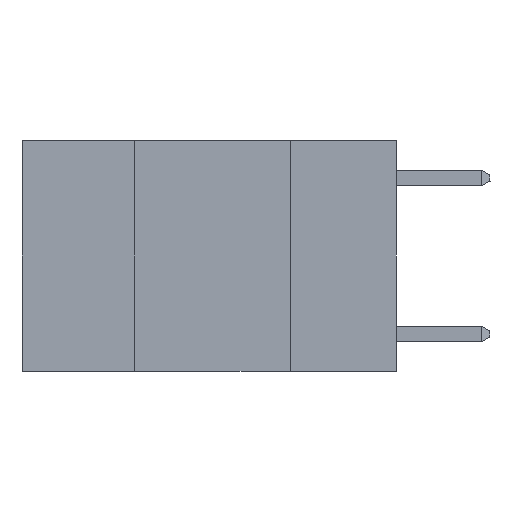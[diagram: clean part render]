
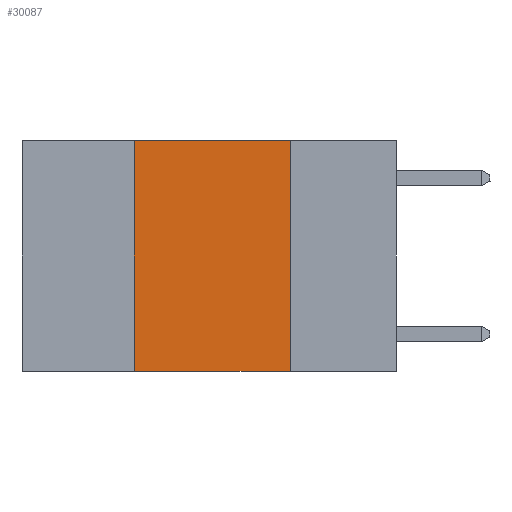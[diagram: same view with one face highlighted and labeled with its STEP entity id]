
A CAD part, left-side view. The second image highlights one B-rep face of the part: STEP entity #30087.
In plain terms, the highlighted planar face has unit normal (-1, 0, 0).
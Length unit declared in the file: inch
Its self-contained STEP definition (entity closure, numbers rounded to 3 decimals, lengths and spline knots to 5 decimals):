
#378 = DIRECTION ( 'NONE',  ( 0., 0., 1. ) ) ;
#1301 = CARTESIAN_POINT ( 'NONE',  ( 0., 0.17, 0. ) ) ;
#1878 = ORIENTED_EDGE ( 'NONE', *, *, #22763, .F. ) ;
#1990 = DIRECTION ( 'NONE',  ( 0., 0., -1. ) ) ;
#2859 = CARTESIAN_POINT ( 'NONE',  ( 0., 0.17, -0.37 ) ) ;
#5022 = CARTESIAN_POINT ( 'NONE',  ( 0., 0.42, 0. ) ) ;
#5112 = VERTEX_POINT ( 'NONE', #1301 ) ;
#5124 = CARTESIAN_POINT ( 'NONE',  ( 0., 0.6, 0. ) ) ;
#5717 = VECTOR ( 'NONE', #8319, 39.37008 ) ;
#6155 = ORIENTED_EDGE ( 'NONE', *, *, #18616, .T. ) ;
#6591 = CARTESIAN_POINT ( 'NONE',  ( 0., 0.6, 0. ) ) ;
#8319 = DIRECTION ( 'NONE',  ( 0., -1., 0. ) ) ;
#8880 = CARTESIAN_POINT ( 'NONE',  ( 0., 0.6, -0.37 ) ) ;
#9042 = VERTEX_POINT ( 'NONE', #2859 ) ;
#10744 = VECTOR ( 'NONE', #1990, 39.37008 ) ;
#12142 = VERTEX_POINT ( 'NONE', #13112 ) ;
#12416 = PLANE ( 'NONE',  #18822 ) ;
#13112 = CARTESIAN_POINT ( 'NONE',  ( 0., 0.42, 0. ) ) ;
#13920 = CARTESIAN_POINT ( 'NONE',  ( 0., 0.17, 0. ) ) ;
#15042 = FACE_OUTER_BOUND ( 'NONE', #21368, .T. ) ;
#15603 = ORIENTED_EDGE ( 'NONE', *, *, #24122, .F. ) ;
#16143 = LINE ( 'NONE', #8880, #29718 ) ;
#18248 = EDGE_CURVE ( 'NONE', #25460, #12142, #24383, .T. ) ;
#18616 = EDGE_CURVE ( 'NONE', #25460, #9042, #16143, .T. ) ;
#18822 = AXIS2_PLACEMENT_3D ( 'NONE', #5124, #29155, #22005 ) ;
#21087 = DIRECTION ( 'NONE',  ( 0., -1., 0. ) ) ;
#21168 = CARTESIAN_POINT ( 'NONE',  ( 0., 0.42, -0.37 ) ) ;
#21368 = EDGE_LOOP ( 'NONE', ( #15603, #1878, #23709, #6155 ) ) ;
#22005 = DIRECTION ( 'NONE',  ( 0., 0., -1. ) ) ;
#22763 = EDGE_CURVE ( 'NONE', #12142, #5112, #27837, .T. ) ;
#23709 = ORIENTED_EDGE ( 'NONE', *, *, #18248, .F. ) ;
#24122 = EDGE_CURVE ( 'NONE', #5112, #9042, #25377, .T. ) ;
#24383 = LINE ( 'NONE', #5022, #26221 ) ;
#25377 = LINE ( 'NONE', #13920, #10744 ) ;
#25460 = VERTEX_POINT ( 'NONE', #21168 ) ;
#26221 = VECTOR ( 'NONE', #378, 39.37008 ) ;
#27837 = LINE ( 'NONE', #6591, #5717 ) ;
#29155 = DIRECTION ( 'NONE',  ( 1., 0., 0. ) ) ;
#29718 = VECTOR ( 'NONE', #21087, 39.37008 ) ;
#30087 = ADVANCED_FACE ( 'NONE', ( #15042 ), #12416, .F. ) ;
